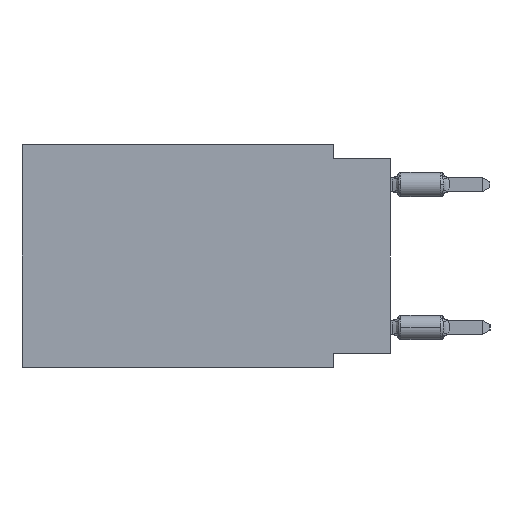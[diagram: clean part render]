
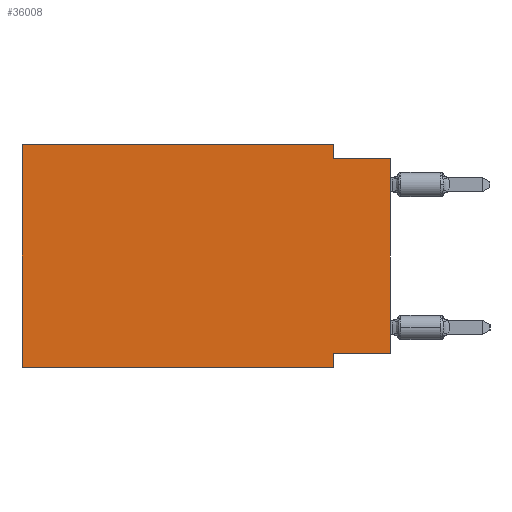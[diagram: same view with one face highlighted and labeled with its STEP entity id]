
A CAD part, left-side view. The second image highlights one B-rep face of the part: STEP entity #36008.
In plain terms, the highlighted planar face has unit normal (-1, 0, 0).
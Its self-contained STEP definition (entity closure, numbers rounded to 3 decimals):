
#380 = VERTEX_POINT ( 'NONE', #27309 ) ;
#1065 = EDGE_CURVE ( 'NONE', #380, #15717, #43259, .T. ) ;
#1569 = VERTEX_POINT ( 'NONE', #8226 ) ;
#3319 = DIRECTION ( 'NONE',  ( 0., -1., 0. ) ) ;
#3820 = VERTEX_POINT ( 'NONE', #33691 ) ;
#5555 = AXIS2_PLACEMENT_3D ( 'NONE', #44630, #13958, #27440 ) ;
#6999 = ORIENTED_EDGE ( 'NONE', *, *, #44502, .F. ) ;
#7230 = CARTESIAN_POINT ( 'NONE',  ( 0., 16.383, -9.906 ) ) ;
#8201 = EDGE_CURVE ( 'NONE', #11229, #33244, #19261, .T. ) ;
#8226 = CARTESIAN_POINT ( 'NONE',  ( 0., 2.54, -9.271 ) ) ;
#8598 = VECTOR ( 'NONE', #43038, 1000. ) ;
#8947 = LINE ( 'NONE', #16039, #24714 ) ;
#9773 = ORIENTED_EDGE ( 'NONE', *, *, #17110, .T. ) ;
#11229 = VERTEX_POINT ( 'NONE', #20026 ) ;
#11909 = DIRECTION ( 'NONE',  ( 0., -1., 0. ) ) ;
#11958 = DIRECTION ( 'NONE',  ( 0., 0., 1. ) ) ;
#13061 = PLANE ( 'NONE',  #5555 ) ;
#13878 = ORIENTED_EDGE ( 'NONE', *, *, #45050, .F. ) ;
#13958 = DIRECTION ( 'NONE',  ( 1., 0., 0. ) ) ;
#14171 = VERTEX_POINT ( 'NONE', #44558 ) ;
#14552 = EDGE_CURVE ( 'NONE', #14171, #11229, #33455, .T. ) ;
#14553 = ORIENTED_EDGE ( 'NONE', *, *, #38133, .F. ) ;
#15259 = VECTOR ( 'NONE', #43194, 1000. ) ;
#15717 = VERTEX_POINT ( 'NONE', #25751 ) ;
#16039 = CARTESIAN_POINT ( 'NONE',  ( 0., 0., -0.635 ) ) ;
#16052 = CARTESIAN_POINT ( 'NONE',  ( 0., 0., 0. ) ) ;
#16525 = DIRECTION ( 'NONE',  ( 0., -1., 0. ) ) ;
#16899 = VECTOR ( 'NONE', #36833, 1000. ) ;
#17110 = EDGE_CURVE ( 'NONE', #14171, #3820, #24834, .T. ) ;
#18979 = VECTOR ( 'NONE', #30901, 1000. ) ;
#19159 = CARTESIAN_POINT ( 'NONE',  ( 0., 2.54, -9.906 ) ) ;
#19261 = LINE ( 'NONE', #26586, #42312 ) ;
#20026 = CARTESIAN_POINT ( 'NONE',  ( 0., 16.383, 0. ) ) ;
#20834 = CARTESIAN_POINT ( 'NONE',  ( 0., 0., -9.271 ) ) ;
#20837 = VECTOR ( 'NONE', #3319, 1000. ) ;
#24714 = VECTOR ( 'NONE', #11909, 1000. ) ;
#24834 = LINE ( 'NONE', #7230, #20837 ) ;
#25751 = CARTESIAN_POINT ( 'NONE',  ( 0., 0., -0.635 ) ) ;
#25769 = VECTOR ( 'NONE', #11958, 1000. ) ;
#26586 = CARTESIAN_POINT ( 'NONE',  ( 0., 16.383, 0. ) ) ;
#26591 = CARTESIAN_POINT ( 'NONE',  ( 0., 16.383, 0. ) ) ;
#26976 = ORIENTED_EDGE ( 'NONE', *, *, #27734, .F. ) ;
#27309 = CARTESIAN_POINT ( 'NONE',  ( 0., 0., -9.271 ) ) ;
#27440 = DIRECTION ( 'NONE',  ( 0., 0., -1. ) ) ;
#27734 = EDGE_CURVE ( 'NONE', #44214, #15717, #8947, .T. ) ;
#28700 = ORIENTED_EDGE ( 'NONE', *, *, #14552, .F. ) ;
#30901 = DIRECTION ( 'NONE',  ( 0., 1., 0. ) ) ;
#33166 = CARTESIAN_POINT ( 'NONE',  ( 0., 2.54, 0. ) ) ;
#33244 = VERTEX_POINT ( 'NONE', #35289 ) ;
#33455 = LINE ( 'NONE', #26591, #25769 ) ;
#33651 = FACE_OUTER_BOUND ( 'NONE', #42557, .T. ) ;
#33691 = CARTESIAN_POINT ( 'NONE',  ( 0., 2.54, -9.906 ) ) ;
#35289 = CARTESIAN_POINT ( 'NONE',  ( 0., 2.54, 0. ) ) ;
#35448 = ORIENTED_EDGE ( 'NONE', *, *, #8201, .F. ) ;
#36008 = ADVANCED_FACE ( 'NONE', ( #33651 ), #13061, .F. ) ;
#36311 = LINE ( 'NONE', #19159, #15259 ) ;
#36833 = DIRECTION ( 'NONE',  ( 0., 0., 1. ) ) ;
#38133 = EDGE_CURVE ( 'NONE', #33244, #44214, #40494, .T. ) ;
#40494 = LINE ( 'NONE', #33166, #8598 ) ;
#41428 = LINE ( 'NONE', #20834, #18979 ) ;
#42312 = VECTOR ( 'NONE', #16525, 1000. ) ;
#42557 = EDGE_LOOP ( 'NONE', ( #43388, #26976, #14553, #35448, #28700, #9773, #13878, #6999 ) ) ;
#43038 = DIRECTION ( 'NONE',  ( 0., 0., -1. ) ) ;
#43075 = CARTESIAN_POINT ( 'NONE',  ( 0., 2.54, -0.635 ) ) ;
#43194 = DIRECTION ( 'NONE',  ( 0., 0., -1. ) ) ;
#43259 = LINE ( 'NONE', #16052, #16899 ) ;
#43388 = ORIENTED_EDGE ( 'NONE', *, *, #1065, .T. ) ;
#44214 = VERTEX_POINT ( 'NONE', #43075 ) ;
#44502 = EDGE_CURVE ( 'NONE', #380, #1569, #41428, .T. ) ;
#44558 = CARTESIAN_POINT ( 'NONE',  ( 0., 16.383, -9.906 ) ) ;
#44630 = CARTESIAN_POINT ( 'NONE',  ( 0., 16.383, 0. ) ) ;
#45050 = EDGE_CURVE ( 'NONE', #1569, #3820, #36311, .T. ) ;
